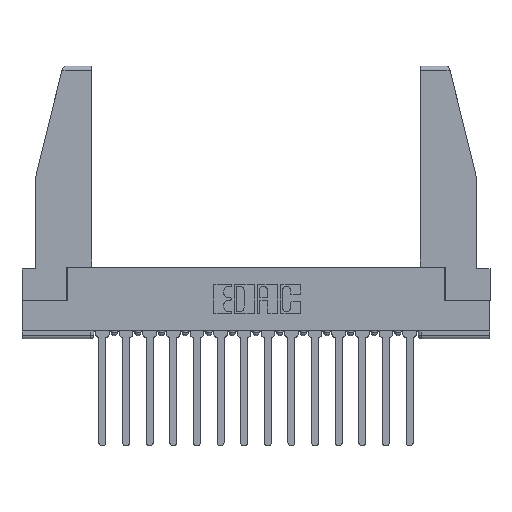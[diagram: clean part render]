
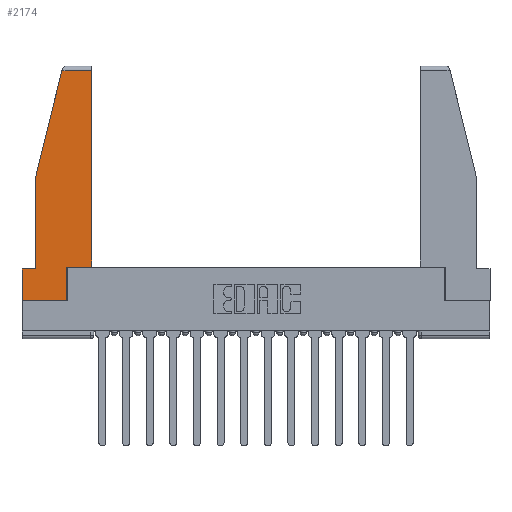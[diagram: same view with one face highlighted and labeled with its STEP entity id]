
A CAD part, top view. The second image highlights one B-rep face of the part: STEP entity #2174.
In plain terms, the highlighted planar face has unit normal (0, 0, 1).
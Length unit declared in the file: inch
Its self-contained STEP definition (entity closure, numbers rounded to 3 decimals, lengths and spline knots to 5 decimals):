
#4 = LINE ( 'NONE', #5278, #9392 ) ;
#289 = VECTOR ( 'NONE', #2765, 39.37008 ) ;
#408 = LINE ( 'NONE', #15433, #16354 ) ;
#447 = ORIENTED_EDGE ( 'NONE', *, *, #6142, .T. ) ;
#824 = CARTESIAN_POINT ( 'NONE',  ( 0.297, 0.223, 0. ) ) ;
#1005 = ORIENTED_EDGE ( 'NONE', *, *, #12173, .T. ) ;
#1095 = ORIENTED_EDGE ( 'NONE', *, *, #1240, .T. ) ;
#1177 = CARTESIAN_POINT ( 'NONE',  ( 0., 0., 0. ) ) ;
#1196 = CARTESIAN_POINT ( 'NONE',  ( 0.086, 0.8, 0. ) ) ;
#1240 = EDGE_CURVE ( 'NONE', #13151, #9897, #8117, .T. ) ;
#1335 = CARTESIAN_POINT ( 'NONE',  ( 0.297, 0., 0. ) ) ;
#1392 = EDGE_CURVE ( 'NONE', #3761, #13329, #7276, .T. ) ;
#1645 = VERTEX_POINT ( 'NONE', #3684 ) ;
#1809 = CARTESIAN_POINT ( 'NONE',  ( 0.086, 0.21, 0. ) ) ;
#2022 = VECTOR ( 'NONE', #3851, 39.37008 ) ;
#2174 = ADVANCED_FACE ( 'NONE', ( #12443 ), #11087, .T. ) ;
#2387 = DIRECTION ( 'NONE',  ( 0., 1., 0. ) ) ;
#2765 = DIRECTION ( 'NONE',  ( 1., 0., 0. ) ) ;
#2821 = EDGE_LOOP ( 'NONE', ( #447, #1005, #11838, #17563, #11833, #1095, #14226, #6649, #13014 ) ) ;
#2916 = VERTEX_POINT ( 'NONE', #3261 ) ;
#3039 = DIRECTION ( 'NONE',  ( -1., 0., 0. ) ) ;
#3261 = CARTESIAN_POINT ( 'NONE',  ( 0.086, 0.8, 0. ) ) ;
#3461 = CARTESIAN_POINT ( 'NONE',  ( 0.297, 0., 0. ) ) ;
#3556 = LINE ( 'NONE', #3461, #9258 ) ;
#3684 = CARTESIAN_POINT ( 'NONE',  ( 0.461, 1.52, 0. ) ) ;
#3761 = VERTEX_POINT ( 'NONE', #824 ) ;
#3789 = EDGE_CURVE ( 'NONE', #11602, #3761, #3556, .T. ) ;
#3851 = DIRECTION ( 'NONE',  ( 0., -1., 0. ) ) ;
#3989 = EDGE_CURVE ( 'NONE', #2916, #12977, #6645, .T. ) ;
#4540 = CARTESIAN_POINT ( 'NONE',  ( 0.297, 0.223, 0. ) ) ;
#5144 = VECTOR ( 'NONE', #7968, 39.37008 ) ;
#5254 = CARTESIAN_POINT ( 'NONE',  ( 0., 0., 0. ) ) ;
#5278 = CARTESIAN_POINT ( 'NONE',  ( 0.271, 1.55, 0. ) ) ;
#5372 = LINE ( 'NONE', #10871, #17591 ) ;
#5398 = CARTESIAN_POINT ( 'NONE',  ( 0., 0.21, 0. ) ) ;
#6142 = EDGE_CURVE ( 'NONE', #13329, #1645, #9259, .T. ) ;
#6518 = LINE ( 'NONE', #5254, #5144 ) ;
#6645 = LINE ( 'NONE', #1196, #11005 ) ;
#6649 = ORIENTED_EDGE ( 'NONE', *, *, #3789, .T. ) ;
#6894 = DIRECTION ( 'NONE',  ( -0.239, -0.971, 0. ) ) ;
#7067 = CARTESIAN_POINT ( 'NONE',  ( 0.2636, 1.52, 0. ) ) ;
#7276 = LINE ( 'NONE', #4540, #289 ) ;
#7968 = DIRECTION ( 'NONE',  ( 1., 0., 0. ) ) ;
#8117 = LINE ( 'NONE', #5398, #2022 ) ;
#8375 = DIRECTION ( 'NONE',  ( 1., 0., 0. ) ) ;
#8575 = CARTESIAN_POINT ( 'NONE',  ( 0.461, 0.223, 0. ) ) ;
#9258 = VECTOR ( 'NONE', #14775, 39.37008 ) ;
#9259 = LINE ( 'NONE', #14769, #15271 ) ;
#9392 = VECTOR ( 'NONE', #6894, 39.37008 ) ;
#9897 = VERTEX_POINT ( 'NONE', #1177 ) ;
#9899 = EDGE_CURVE ( 'NONE', #12875, #2916, #4, .T. ) ;
#10871 = CARTESIAN_POINT ( 'NONE',  ( 0., 0.21, 0. ) ) ;
#11005 = VECTOR ( 'NONE', #15138, 39.37008 ) ;
#11087 = PLANE ( 'NONE',  #14347 ) ;
#11602 = VERTEX_POINT ( 'NONE', #1335 ) ;
#11833 = ORIENTED_EDGE ( 'NONE', *, *, #17161, .T. ) ;
#11838 = ORIENTED_EDGE ( 'NONE', *, *, #9899, .T. ) ;
#12173 = EDGE_CURVE ( 'NONE', #1645, #12875, #408, .T. ) ;
#12443 = FACE_OUTER_BOUND ( 'NONE', #2821, .T. ) ;
#12875 = VERTEX_POINT ( 'NONE', #7067 ) ;
#12977 = VERTEX_POINT ( 'NONE', #1809 ) ;
#13014 = ORIENTED_EDGE ( 'NONE', *, *, #1392, .T. ) ;
#13151 = VERTEX_POINT ( 'NONE', #13555 ) ;
#13329 = VERTEX_POINT ( 'NONE', #8575 ) ;
#13555 = CARTESIAN_POINT ( 'NONE',  ( 0., 0.21, 0. ) ) ;
#13684 = DIRECTION ( 'NONE',  ( -1., 0., 0. ) ) ;
#14226 = ORIENTED_EDGE ( 'NONE', *, *, #15630, .T. ) ;
#14347 = AXIS2_PLACEMENT_3D ( 'NONE', #16342, #15239, #8375 ) ;
#14769 = CARTESIAN_POINT ( 'NONE',  ( 0.461, 0.223, 0. ) ) ;
#14775 = DIRECTION ( 'NONE',  ( 0., 1., 0. ) ) ;
#15138 = DIRECTION ( 'NONE',  ( 0., -1., 0. ) ) ;
#15239 = DIRECTION ( 'NONE',  ( 0., 0., 1. ) ) ;
#15271 = VECTOR ( 'NONE', #2387, 39.37008 ) ;
#15433 = CARTESIAN_POINT ( 'NONE',  ( 0., 1.52, 0. ) ) ;
#15630 = EDGE_CURVE ( 'NONE', #9897, #11602, #6518, .T. ) ;
#16342 = CARTESIAN_POINT ( 'NONE',  ( 0., 0., 0. ) ) ;
#16354 = VECTOR ( 'NONE', #3039, 39.37008 ) ;
#17161 = EDGE_CURVE ( 'NONE', #12977, #13151, #5372, .T. ) ;
#17563 = ORIENTED_EDGE ( 'NONE', *, *, #3989, .T. ) ;
#17591 = VECTOR ( 'NONE', #13684, 39.37008 ) ;
